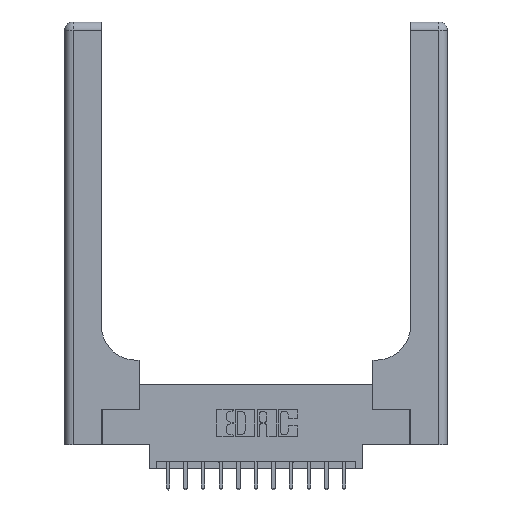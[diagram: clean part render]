
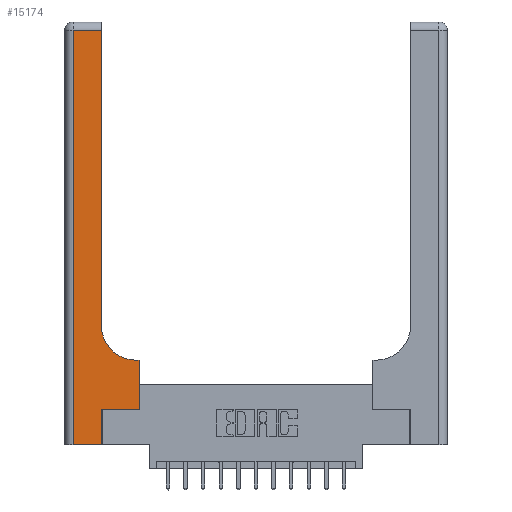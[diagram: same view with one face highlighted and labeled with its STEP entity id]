
A CAD part, top view. The second image highlights one B-rep face of the part: STEP entity #15174.
In plain terms, the highlighted planar face has unit normal (0, 0, 1).
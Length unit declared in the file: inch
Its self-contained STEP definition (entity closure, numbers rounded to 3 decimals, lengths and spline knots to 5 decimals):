
#149 = CARTESIAN_POINT ( 'NONE',  ( 0.51, 0.6, 0.37 ) ) ;
#253 = ORIENTED_EDGE ( 'NONE', *, *, #7305, .T. ) ;
#501 = ORIENTED_EDGE ( 'NONE', *, *, #16565, .T. ) ;
#593 = EDGE_CURVE ( 'NONE', #1869, #12352, #9494, .T. ) ;
#801 = VERTEX_POINT ( 'NONE', #1963 ) ;
#927 = EDGE_CURVE ( 'NONE', #8994, #801, #11490, .T. ) ;
#1154 = EDGE_CURVE ( 'NONE', #801, #4129, #1751, .T. ) ;
#1751 = LINE ( 'NONE', #12150, #15477 ) ;
#1802 = CARTESIAN_POINT ( 'NONE',  ( 0., 0., 0.37 ) ) ;
#1869 = VERTEX_POINT ( 'NONE', #12182 ) ;
#1963 = CARTESIAN_POINT ( 'NONE',  ( 0.528, 0.25, 0.37 ) ) ;
#2046 = DIRECTION ( 'NONE',  ( 0., 1., 0. ) ) ;
#2719 = CARTESIAN_POINT ( 'NONE',  ( 0.265, 0., 0.37 ) ) ;
#3079 = CARTESIAN_POINT ( 'NONE',  ( 0.265, 0., 0.37 ) ) ;
#3666 = VECTOR ( 'NONE', #3998, 39.37008 ) ;
#3998 = DIRECTION ( 'NONE',  ( 0., 1., 0. ) ) ;
#4000 = VECTOR ( 'NONE', #15854, 39.37008 ) ;
#4041 = DIRECTION ( 'NONE',  ( -1., 0., 0. ) ) ;
#4129 = VERTEX_POINT ( 'NONE', #9516 ) ;
#4136 = VERTEX_POINT ( 'NONE', #3079 ) ;
#4308 = EDGE_LOOP ( 'NONE', ( #7783, #9029, #10287, #13027, #13648, #15479, #16584, #253, #501 ) ) ;
#4318 = CARTESIAN_POINT ( 'NONE',  ( 0.26, 0.6, 0.37 ) ) ;
#4326 = CARTESIAN_POINT ( 'NONE',  ( 0.06, 0., 0.37 ) ) ;
#4405 = DIRECTION ( 'NONE',  ( 0., 1., 0. ) ) ;
#4497 = EDGE_CURVE ( 'NONE', #4136, #8994, #10545, .T. ) ;
#4603 = VECTOR ( 'NONE', #5176, 39.37008 ) ;
#4668 = LINE ( 'NONE', #5975, #11556 ) ;
#5145 = AXIS2_PLACEMENT_3D ( 'NONE', #15575, #11786, #4041 ) ;
#5176 = DIRECTION ( 'NONE',  ( 1., 0., 0. ) ) ;
#5394 = VERTEX_POINT ( 'NONE', #11262 ) ;
#5556 = CARTESIAN_POINT ( 'NONE',  ( 0.06, 2.94, 0.37 ) ) ;
#5601 = VECTOR ( 'NONE', #10867, 39.37008 ) ;
#5975 = CARTESIAN_POINT ( 'NONE',  ( 0.26, 3., 0.37 ) ) ;
#6466 = CARTESIAN_POINT ( 'NONE',  ( 0.265, 0.25, 0.37 ) ) ;
#6816 = DIRECTION ( 'NONE',  ( -1., 0., 0. ) ) ;
#6893 = CARTESIAN_POINT ( 'NONE',  ( 0., 2.94, 0.37 ) ) ;
#7305 = EDGE_CURVE ( 'NONE', #4129, #12809, #10482, .T. ) ;
#7371 = LINE ( 'NONE', #8456, #10408 ) ;
#7561 = DIRECTION ( 'NONE',  ( 0., 0., -1. ) ) ;
#7783 = ORIENTED_EDGE ( 'NONE', *, *, #14936, .T. ) ;
#7895 = PLANE ( 'NONE',  #5145 ) ;
#8456 = CARTESIAN_POINT ( 'NONE',  ( 0.06, 3., 0.37 ) ) ;
#8994 = VERTEX_POINT ( 'NONE', #14407 ) ;
#9029 = ORIENTED_EDGE ( 'NONE', *, *, #593, .T. ) ;
#9104 = VERTEX_POINT ( 'NONE', #4326 ) ;
#9494 = LINE ( 'NONE', #6893, #15891 ) ;
#9516 = CARTESIAN_POINT ( 'NONE',  ( 0.528, 0.6, 0.37 ) ) ;
#9772 = DIRECTION ( 'NONE',  ( 0., -1., 0. ) ) ;
#10287 = ORIENTED_EDGE ( 'NONE', *, *, #13058, .T. ) ;
#10408 = VECTOR ( 'NONE', #9772, 39.37008 ) ;
#10482 = LINE ( 'NONE', #4318, #4000 ) ;
#10545 = LINE ( 'NONE', #2719, #3666 ) ;
#10774 = AXIS2_PLACEMENT_3D ( 'NONE', #15252, #7561, #16499 ) ;
#10867 = DIRECTION ( 'NONE',  ( 1., 0., 0. ) ) ;
#11262 = CARTESIAN_POINT ( 'NONE',  ( 0.26, 0.85, 0.37 ) ) ;
#11490 = LINE ( 'NONE', #6466, #4603 ) ;
#11556 = VECTOR ( 'NONE', #2046, 39.37008 ) ;
#11786 = DIRECTION ( 'NONE',  ( 0., 0., -1. ) ) ;
#11955 = EDGE_CURVE ( 'NONE', #9104, #4136, #12042, .T. ) ;
#12042 = LINE ( 'NONE', #1802, #5601 ) ;
#12150 = CARTESIAN_POINT ( 'NONE',  ( 0.528, 0.25, 0.37 ) ) ;
#12182 = CARTESIAN_POINT ( 'NONE',  ( 0.26, 2.94, 0.37 ) ) ;
#12352 = VERTEX_POINT ( 'NONE', #5556 ) ;
#12809 = VERTEX_POINT ( 'NONE', #149 ) ;
#13027 = ORIENTED_EDGE ( 'NONE', *, *, #11955, .T. ) ;
#13058 = EDGE_CURVE ( 'NONE', #12352, #9104, #7371, .T. ) ;
#13648 = ORIENTED_EDGE ( 'NONE', *, *, #4497, .T. ) ;
#14372 = FACE_OUTER_BOUND ( 'NONE', #4308, .T. ) ;
#14407 = CARTESIAN_POINT ( 'NONE',  ( 0.265, 0.25, 0.37 ) ) ;
#14936 = EDGE_CURVE ( 'NONE', #5394, #1869, #4668, .T. ) ;
#15174 = ADVANCED_FACE ( 'NONE', ( #14372 ), #7895, .F. ) ;
#15252 = CARTESIAN_POINT ( 'NONE',  ( 0.51, 0.85, 0.37 ) ) ;
#15477 = VECTOR ( 'NONE', #4405, 39.37008 ) ;
#15479 = ORIENTED_EDGE ( 'NONE', *, *, #927, .T. ) ;
#15575 = CARTESIAN_POINT ( 'NONE',  ( 0., 3., 0.37 ) ) ;
#15854 = DIRECTION ( 'NONE',  ( -1., 0., 0. ) ) ;
#15891 = VECTOR ( 'NONE', #6816, 39.37008 ) ;
#16307 = CIRCLE ( 'NONE', #10774, 0.25 ) ;
#16499 = DIRECTION ( 'NONE',  ( 1., 0., 0. ) ) ;
#16565 = EDGE_CURVE ( 'NONE', #12809, #5394, #16307, .T. ) ;
#16584 = ORIENTED_EDGE ( 'NONE', *, *, #1154, .T. ) ;
